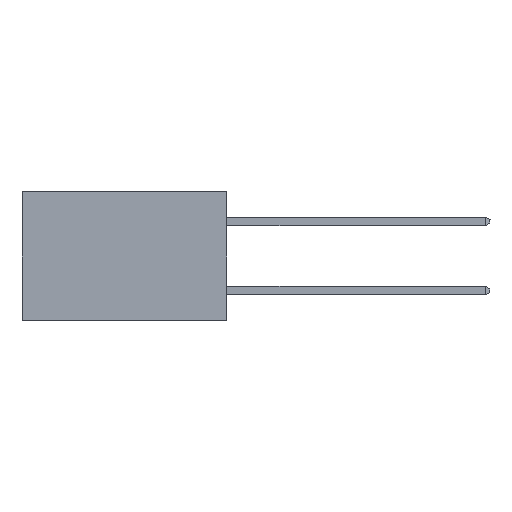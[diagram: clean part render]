
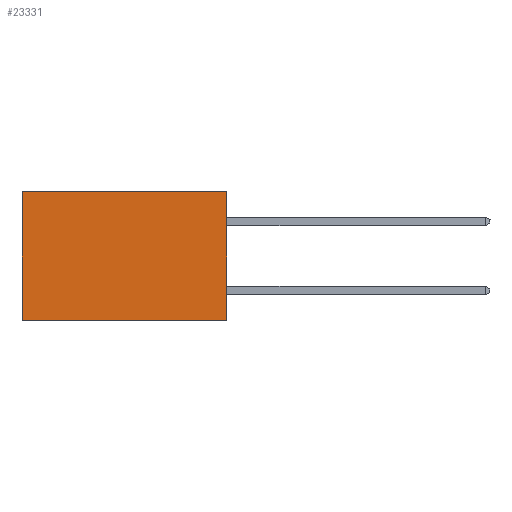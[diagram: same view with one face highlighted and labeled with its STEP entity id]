
A CAD part, left-side view. The second image highlights one B-rep face of the part: STEP entity #23331.
In plain terms, the highlighted planar face has unit normal (-1, 0, 0).
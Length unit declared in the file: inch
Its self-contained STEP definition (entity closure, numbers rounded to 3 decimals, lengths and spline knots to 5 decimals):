
#27 = EDGE_CURVE ( 'NONE', #1566, #24538, #19286, .T. ) ;
#157 = DIRECTION ( 'NONE',  ( 0., 0., -1. ) ) ;
#1566 = VERTEX_POINT ( 'NONE', #17671 ) ;
#2862 = ORIENTED_EDGE ( 'NONE', *, *, #23550, .T. ) ;
#3064 = CARTESIAN_POINT ( 'NONE',  ( 0.277, 0., -0.37 ) ) ;
#7480 = LINE ( 'NONE', #10611, #27044 ) ;
#7953 = EDGE_CURVE ( 'NONE', #8761, #1566, #7480, .T. ) ;
#8761 = VERTEX_POINT ( 'NONE', #22665 ) ;
#9830 = DIRECTION ( 'NONE',  ( 0., 0., -1. ) ) ;
#10611 = CARTESIAN_POINT ( 'NONE',  ( 0.277, 0., -0.37 ) ) ;
#11372 = ORIENTED_EDGE ( 'NONE', *, *, #27, .F. ) ;
#11841 = LINE ( 'NONE', #23985, #32082 ) ;
#13129 = PLANE ( 'NONE',  #22686 ) ;
#14211 = LINE ( 'NONE', #28285, #18581 ) ;
#14644 = ORIENTED_EDGE ( 'NONE', *, *, #7953, .F. ) ;
#15701 = DIRECTION ( 'NONE',  ( 1., 0., 0. ) ) ;
#17655 = CARTESIAN_POINT ( 'NONE',  ( 0.277, 0.59, -0.37 ) ) ;
#17671 = CARTESIAN_POINT ( 'NONE',  ( 0.277, 0., -0.37 ) ) ;
#18581 = VECTOR ( 'NONE', #30815, 39.37008 ) ;
#19286 = LINE ( 'NONE', #3064, #31892 ) ;
#20521 = VERTEX_POINT ( 'NONE', #26570 ) ;
#22665 = CARTESIAN_POINT ( 'NONE',  ( 0.277, 0., 0. ) ) ;
#22686 = AXIS2_PLACEMENT_3D ( 'NONE', #30831, #15701, #157 ) ;
#23331 = ADVANCED_FACE ( 'NONE', ( #25000 ), #13129, .F. ) ;
#23550 = EDGE_CURVE ( 'NONE', #20521, #24538, #11841, .T. ) ;
#23985 = CARTESIAN_POINT ( 'NONE',  ( 0.277, 0.59, -0.37 ) ) ;
#24538 = VERTEX_POINT ( 'NONE', #17655 ) ;
#25000 = FACE_OUTER_BOUND ( 'NONE', #26405, .T. ) ;
#26405 = EDGE_LOOP ( 'NONE', ( #2862, #11372, #14644, #29675 ) ) ;
#26539 = DIRECTION ( 'NONE',  ( 0., 0., -1. ) ) ;
#26570 = CARTESIAN_POINT ( 'NONE',  ( 0.277, 0.59, 0. ) ) ;
#26896 = DIRECTION ( 'NONE',  ( 0., 1., 0. ) ) ;
#27044 = VECTOR ( 'NONE', #9830, 39.37008 ) ;
#28285 = CARTESIAN_POINT ( 'NONE',  ( 0.277, 0., 0. ) ) ;
#29675 = ORIENTED_EDGE ( 'NONE', *, *, #30521, .T. ) ;
#30521 = EDGE_CURVE ( 'NONE', #8761, #20521, #14211, .T. ) ;
#30815 = DIRECTION ( 'NONE',  ( 0., 1., 0. ) ) ;
#30831 = CARTESIAN_POINT ( 'NONE',  ( 0.277, 0., -0.37 ) ) ;
#31892 = VECTOR ( 'NONE', #26896, 39.37008 ) ;
#32082 = VECTOR ( 'NONE', #26539, 39.37008 ) ;
